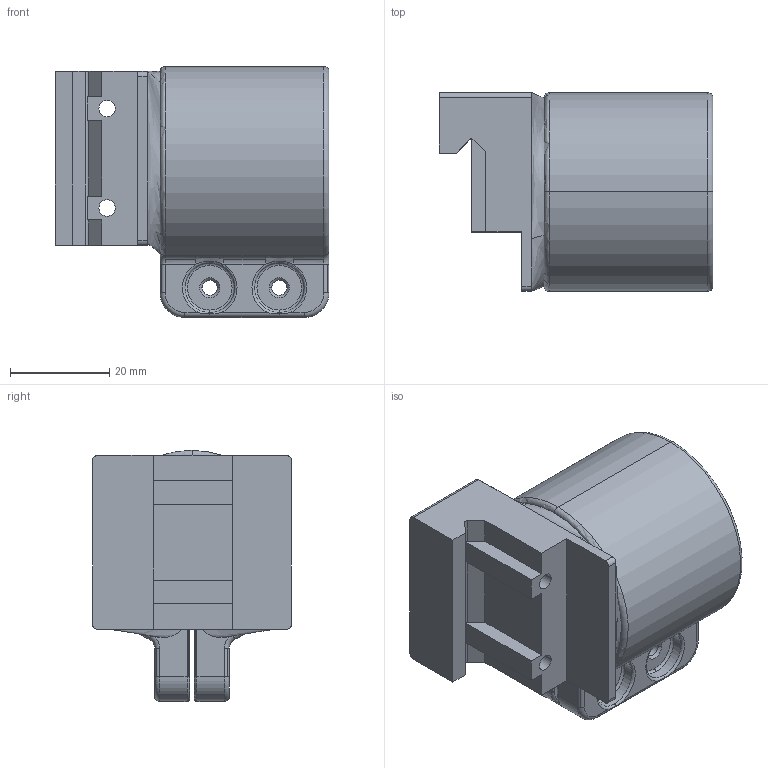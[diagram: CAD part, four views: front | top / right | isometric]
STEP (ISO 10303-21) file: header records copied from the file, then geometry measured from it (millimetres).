
FILE_DESCRIPTION (( 'STEP AP203' ), '1' );
FILE_NAME ('AR Buffer Tube Rail Adapter.STEP', '2020-10-26T17:26:23', ( '' ), ( '' ), 'SwSTEP 2.0', 'SolidWorks 2019', '' );
FILE_SCHEMA (( 'CONFIG_CONTROL_DESIGN' ));
Length unit declared in the file: inch
Products named in the file (1): AR Buffer Tube Rail Adapter
Bounding box: 55.14 x 40 x 50.54 mm (x, y, z)
Volume: 43254.1 mm3; surface area: 17030.7 mm2
Topology: 1 solids, 1 shells, 287 faces, 796 edges, 509 vertices
Faces by surface type: cylinder 142, plane 63, bspline 46, torus 26, cone 10
Entity records: 14922 total; most frequent: CARTESIAN_POINT 8042, ORIENTED_EDGE 1588, DIRECTION 1187, EDGE_CURVE 794, VERTEX_POINT 509, AXIS2_PLACEMENT_3D 428, LINE 331, VECTOR 331
